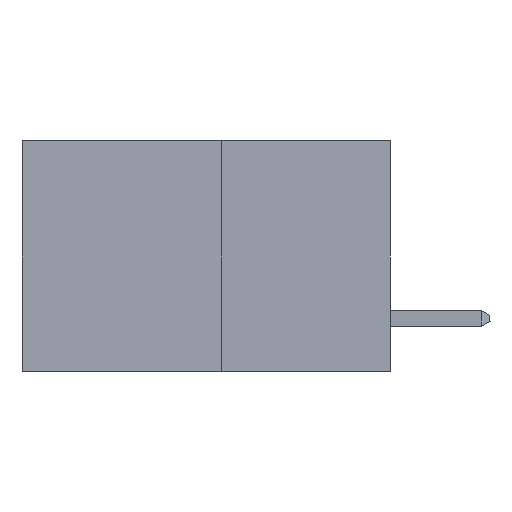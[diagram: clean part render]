
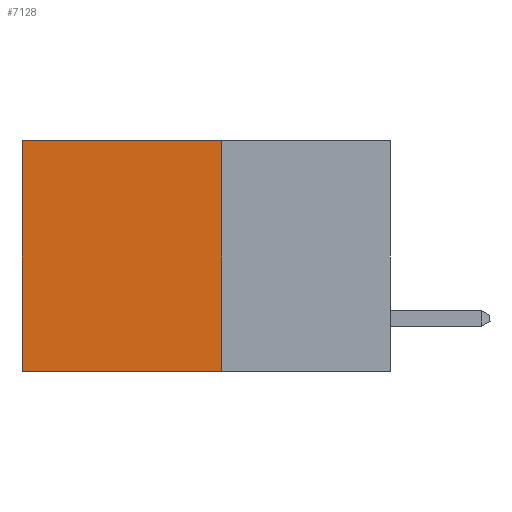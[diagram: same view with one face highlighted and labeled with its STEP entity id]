
A CAD part, left-side view. The second image highlights one B-rep face of the part: STEP entity #7128.
In plain terms, the highlighted planar face has unit normal (-1, 0, 0).
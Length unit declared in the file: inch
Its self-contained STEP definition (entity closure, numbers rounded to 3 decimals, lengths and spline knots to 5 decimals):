
#893 = CARTESIAN_POINT ( 'NONE',  ( 0.277, 0.27, -0.37 ) ) ;
#1293 = CARTESIAN_POINT ( 'NONE',  ( 0.277, 0.59, 0. ) ) ;
#3640 = EDGE_CURVE ( 'NONE', #4778, #13997, #12538, .T. ) ;
#3671 = LINE ( 'NONE', #12163, #9713 ) ;
#4271 = CARTESIAN_POINT ( 'NONE',  ( 0.277, 0.59, -0.37 ) ) ;
#4278 = DIRECTION ( 'NONE',  ( 0., 1., 0. ) ) ;
#4778 = VERTEX_POINT ( 'NONE', #893 ) ;
#5257 = ORIENTED_EDGE ( 'NONE', *, *, #11843, .F. ) ;
#5680 = AXIS2_PLACEMENT_3D ( 'NONE', #6211, #12617, #13906 ) ;
#5929 = VECTOR ( 'NONE', #13560, 39.37008 ) ;
#6211 = CARTESIAN_POINT ( 'NONE',  ( 0.277, 0.27, -0.37 ) ) ;
#6400 = VERTEX_POINT ( 'NONE', #8753 ) ;
#6600 = CARTESIAN_POINT ( 'NONE',  ( 0.277, 0.59, -0.37 ) ) ;
#6762 = VECTOR ( 'NONE', #12158, 39.37008 ) ;
#6897 = CARTESIAN_POINT ( 'NONE',  ( 0.277, 0.27, -0.37 ) ) ;
#6947 = DIRECTION ( 'NONE',  ( 0., 1., 0. ) ) ;
#6949 = VECTOR ( 'NONE', #6947, 39.37008 ) ;
#7128 = ADVANCED_FACE ( 'NONE', ( #8839 ), #12411, .F. ) ;
#8263 = ORIENTED_EDGE ( 'NONE', *, *, #3640, .F. ) ;
#8753 = CARTESIAN_POINT ( 'NONE',  ( 0.277, 0.27, 0. ) ) ;
#8839 = FACE_OUTER_BOUND ( 'NONE', #12634, .T. ) ;
#9430 = LINE ( 'NONE', #4271, #6762 ) ;
#9713 = VECTOR ( 'NONE', #4278, 39.37008 ) ;
#10240 = ORIENTED_EDGE ( 'NONE', *, *, #13353, .T. ) ;
#10326 = CARTESIAN_POINT ( 'NONE',  ( 0.277, 0.27, -0.37 ) ) ;
#10454 = EDGE_CURVE ( 'NONE', #6400, #12485, #3671, .T. ) ;
#11306 = ORIENTED_EDGE ( 'NONE', *, *, #10454, .T. ) ;
#11608 = LINE ( 'NONE', #10326, #5929 ) ;
#11843 = EDGE_CURVE ( 'NONE', #6400, #4778, #11608, .T. ) ;
#12158 = DIRECTION ( 'NONE',  ( 0., 0., -1. ) ) ;
#12163 = CARTESIAN_POINT ( 'NONE',  ( 0.277, 0.27, 0. ) ) ;
#12411 = PLANE ( 'NONE',  #5680 ) ;
#12485 = VERTEX_POINT ( 'NONE', #1293 ) ;
#12538 = LINE ( 'NONE', #6897, #6949 ) ;
#12617 = DIRECTION ( 'NONE',  ( 1., 0., 0. ) ) ;
#12634 = EDGE_LOOP ( 'NONE', ( #10240, #8263, #5257, #11306 ) ) ;
#13353 = EDGE_CURVE ( 'NONE', #12485, #13997, #9430, .T. ) ;
#13560 = DIRECTION ( 'NONE',  ( 0., 0., -1. ) ) ;
#13906 = DIRECTION ( 'NONE',  ( 0., 0., -1. ) ) ;
#13997 = VERTEX_POINT ( 'NONE', #6600 ) ;
